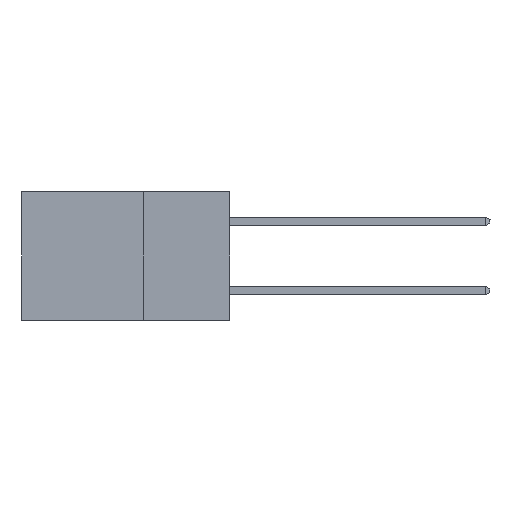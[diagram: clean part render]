
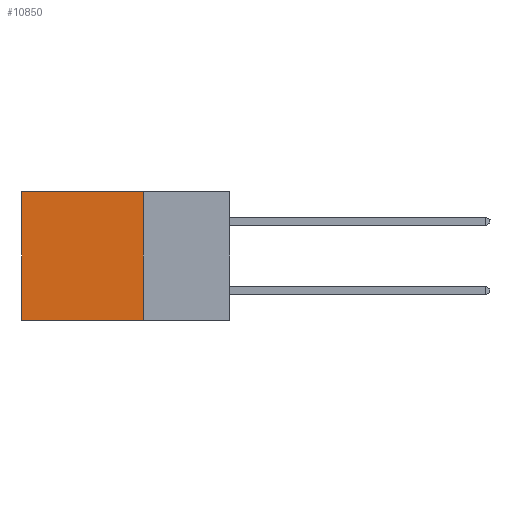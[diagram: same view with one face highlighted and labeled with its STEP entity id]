
A CAD part, left-side view. The second image highlights one B-rep face of the part: STEP entity #10850.
In plain terms, the highlighted planar face has unit normal (-1, 0, 0).
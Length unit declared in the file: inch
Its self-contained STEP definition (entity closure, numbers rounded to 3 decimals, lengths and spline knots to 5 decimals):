
#406 = CARTESIAN_POINT ( 'NONE',  ( 0.298, 0.25, 0. ) ) ;
#931 = EDGE_CURVE ( 'NONE', #1929, #11422, #12270, .T. ) ;
#1031 = CARTESIAN_POINT ( 'NONE',  ( 0.298, 0.25, 0. ) ) ;
#1929 = VERTEX_POINT ( 'NONE', #17020 ) ;
#2040 = VECTOR ( 'NONE', #17435, 39.37008 ) ;
#3637 = EDGE_CURVE ( 'NONE', #7641, #13369, #10304, .T. ) ;
#3836 = EDGE_CURVE ( 'NONE', #11422, #13369, #10523, .T. ) ;
#3990 = EDGE_LOOP ( 'NONE', ( #15234, #14617, #16142, #15208 ) ) ;
#5260 = VECTOR ( 'NONE', #7851, 39.37008 ) ;
#5576 = VECTOR ( 'NONE', #12655, 39.37008 ) ;
#5789 = FACE_OUTER_BOUND ( 'NONE', #3990, .T. ) ;
#6153 = CARTESIAN_POINT ( 'NONE',  ( 0.298, 0.25, -0.37 ) ) ;
#6596 = CARTESIAN_POINT ( 'NONE',  ( 0.298, 0.6, -0.37 ) ) ;
#6747 = CARTESIAN_POINT ( 'NONE',  ( 0.298, 0.25, 0. ) ) ;
#6756 = AXIS2_PLACEMENT_3D ( 'NONE', #6747, #8066, #14702 ) ;
#7641 = VERTEX_POINT ( 'NONE', #9681 ) ;
#7851 = DIRECTION ( 'NONE',  ( 0., 1., 0. ) ) ;
#7875 = CARTESIAN_POINT ( 'NONE',  ( 0.298, 0.6, 0. ) ) ;
#7894 = PLANE ( 'NONE',  #6756 ) ;
#8066 = DIRECTION ( 'NONE',  ( 1., 0., 0. ) ) ;
#9606 = LINE ( 'NONE', #406, #5576 ) ;
#9681 = CARTESIAN_POINT ( 'NONE',  ( 0.298, 0.25, -0.37 ) ) ;
#10304 = LINE ( 'NONE', #6153, #14807 ) ;
#10523 = LINE ( 'NONE', #7875, #2040 ) ;
#10850 = ADVANCED_FACE ( 'NONE', ( #5789 ), #7894, .F. ) ;
#11422 = VERTEX_POINT ( 'NONE', #15831 ) ;
#12270 = LINE ( 'NONE', #1031, #5260 ) ;
#12655 = DIRECTION ( 'NONE',  ( 0., 0., -1. ) ) ;
#13369 = VERTEX_POINT ( 'NONE', #6596 ) ;
#14617 = ORIENTED_EDGE ( 'NONE', *, *, #3637, .F. ) ;
#14702 = DIRECTION ( 'NONE',  ( 0., 0., -1. ) ) ;
#14807 = VECTOR ( 'NONE', #15875, 39.37008 ) ;
#15208 = ORIENTED_EDGE ( 'NONE', *, *, #931, .T. ) ;
#15234 = ORIENTED_EDGE ( 'NONE', *, *, #3836, .T. ) ;
#15831 = CARTESIAN_POINT ( 'NONE',  ( 0.298, 0.6, 0. ) ) ;
#15875 = DIRECTION ( 'NONE',  ( 0., 1., 0. ) ) ;
#16142 = ORIENTED_EDGE ( 'NONE', *, *, #17356, .F. ) ;
#17020 = CARTESIAN_POINT ( 'NONE',  ( 0.298, 0.25, 0. ) ) ;
#17356 = EDGE_CURVE ( 'NONE', #1929, #7641, #9606, .T. ) ;
#17435 = DIRECTION ( 'NONE',  ( 0., 0., -1. ) ) ;
